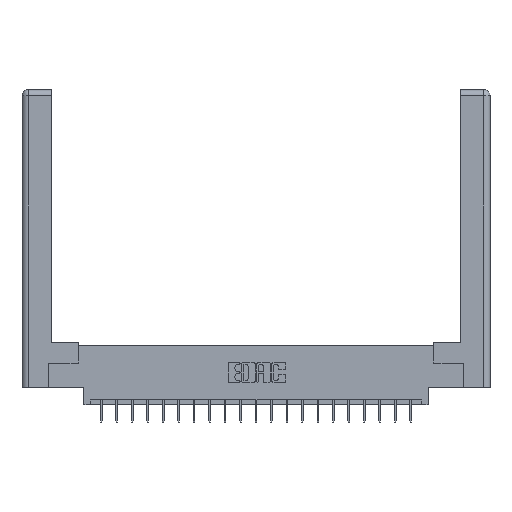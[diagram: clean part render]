
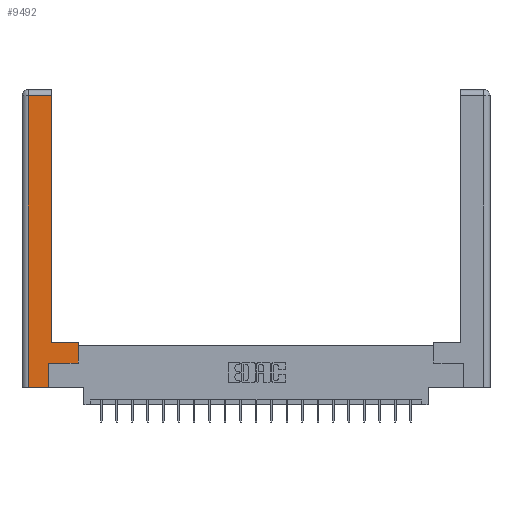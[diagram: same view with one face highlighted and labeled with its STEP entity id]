
A CAD part, top view. The second image highlights one B-rep face of the part: STEP entity #9492.
In plain terms, the highlighted planar face has unit normal (0, 0, 1).
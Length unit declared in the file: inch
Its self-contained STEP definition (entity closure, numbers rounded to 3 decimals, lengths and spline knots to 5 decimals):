
#692 = ORIENTED_EDGE ( 'NONE', *, *, #14860, .T. ) ;
#782 = EDGE_LOOP ( 'NONE', ( #16485, #2539, #20749, #16274, #4995, #19639, #21707, #692 ) ) ;
#1170 = VECTOR ( 'NONE', #1646, 39.37008 ) ;
#1510 = DIRECTION ( 'NONE',  ( 0., 1., 0. ) ) ;
#1646 = DIRECTION ( 'NONE',  ( 0., 1., 0. ) ) ;
#2276 = CARTESIAN_POINT ( 'NONE',  ( 0.565, 0.45, 0. ) ) ;
#2539 = ORIENTED_EDGE ( 'NONE', *, *, #13917, .T. ) ;
#2809 = EDGE_CURVE ( 'NONE', #17671, #3995, #18349, .T. ) ;
#3052 = CARTESIAN_POINT ( 'NONE',  ( 0.565, 0.45, 0. ) ) ;
#3995 = VERTEX_POINT ( 'NONE', #11574 ) ;
#4002 = DIRECTION ( 'NONE',  ( 1., 0., 0. ) ) ;
#4779 = EDGE_CURVE ( 'NONE', #21580, #12341, #20707, .T. ) ;
#4995 = ORIENTED_EDGE ( 'NONE', *, *, #2809, .T. ) ;
#5110 = VERTEX_POINT ( 'NONE', #9535 ) ;
#6011 = CARTESIAN_POINT ( 'NONE',  ( 0., 0., 0. ) ) ;
#6111 = CARTESIAN_POINT ( 'NONE',  ( 0.265, 0.245, 0. ) ) ;
#6197 = CARTESIAN_POINT ( 'NONE',  ( 0.0615, 2.94, 0. ) ) ;
#7934 = DIRECTION ( 'NONE',  ( 0., 1., 0. ) ) ;
#8126 = VERTEX_POINT ( 'NONE', #19199 ) ;
#8534 = LINE ( 'NONE', #13625, #19626 ) ;
#8620 = FACE_OUTER_BOUND ( 'NONE', #782, .T. ) ;
#9492 = ADVANCED_FACE ( 'NONE', ( #8620 ), #19507, .F. ) ;
#9535 = CARTESIAN_POINT ( 'NONE',  ( 0.295, 0.45, 0. ) ) ;
#10474 = VECTOR ( 'NONE', #17544, 39.37008 ) ;
#10750 = LINE ( 'NONE', #17470, #10474 ) ;
#11574 = CARTESIAN_POINT ( 'NONE',  ( 0.265, 0.245, 0. ) ) ;
#11628 = CARTESIAN_POINT ( 'NONE',  ( 0.295, 3., 0. ) ) ;
#11788 = VERTEX_POINT ( 'NONE', #6197 ) ;
#12341 = VERTEX_POINT ( 'NONE', #2276 ) ;
#12623 = VECTOR ( 'NONE', #17944, 39.37008 ) ;
#13130 = VECTOR ( 'NONE', #1510, 39.37008 ) ;
#13625 = CARTESIAN_POINT ( 'NONE',  ( 0.295, 0.45, 0. ) ) ;
#13877 = VECTOR ( 'NONE', #7934, 39.37008 ) ;
#13917 = EDGE_CURVE ( 'NONE', #18769, #11788, #18325, .T. ) ;
#14104 = CARTESIAN_POINT ( 'NONE',  ( 0.0615, 0., 0. ) ) ;
#14414 = AXIS2_PLACEMENT_3D ( 'NONE', #6011, #15960, #16260 ) ;
#14810 = DIRECTION ( 'NONE',  ( -1., 0., 0. ) ) ;
#14860 = EDGE_CURVE ( 'NONE', #12341, #5110, #8534, .T. ) ;
#15720 = VECTOR ( 'NONE', #14810, 39.37008 ) ;
#15960 = DIRECTION ( 'NONE',  ( 0., 0., -1. ) ) ;
#16260 = DIRECTION ( 'NONE',  ( -1., 0., 0. ) ) ;
#16274 = ORIENTED_EDGE ( 'NONE', *, *, #21083, .T. ) ;
#16485 = ORIENTED_EDGE ( 'NONE', *, *, #20163, .T. ) ;
#17470 = CARTESIAN_POINT ( 'NONE',  ( 0.265, 0., 0. ) ) ;
#17544 = DIRECTION ( 'NONE',  ( 1., 0., 0. ) ) ;
#17558 = CARTESIAN_POINT ( 'NONE',  ( 0.565, 0.245, 0. ) ) ;
#17570 = CARTESIAN_POINT ( 'NONE',  ( 0.565, 0.245, 0. ) ) ;
#17671 = VERTEX_POINT ( 'NONE', #18362 ) ;
#17944 = DIRECTION ( 'NONE',  ( 0., -1., 0. ) ) ;
#17969 = EDGE_CURVE ( 'NONE', #3995, #21580, #18474, .T. ) ;
#18124 = CARTESIAN_POINT ( 'NONE',  ( 0.295, 2.94, 0. ) ) ;
#18163 = LINE ( 'NONE', #14104, #12623 ) ;
#18325 = LINE ( 'NONE', #21716, #15720 ) ;
#18349 = LINE ( 'NONE', #6111, #13877 ) ;
#18362 = CARTESIAN_POINT ( 'NONE',  ( 0.265, 0., 0. ) ) ;
#18474 = LINE ( 'NONE', #17558, #20334 ) ;
#18769 = VERTEX_POINT ( 'NONE', #18124 ) ;
#19049 = EDGE_CURVE ( 'NONE', #11788, #8126, #18163, .T. ) ;
#19199 = CARTESIAN_POINT ( 'NONE',  ( 0.0615, 0., 0. ) ) ;
#19507 = PLANE ( 'NONE',  #14414 ) ;
#19626 = VECTOR ( 'NONE', #20414, 39.37008 ) ;
#19639 = ORIENTED_EDGE ( 'NONE', *, *, #17969, .T. ) ;
#20163 = EDGE_CURVE ( 'NONE', #5110, #18769, #20802, .T. ) ;
#20334 = VECTOR ( 'NONE', #4002, 39.37008 ) ;
#20414 = DIRECTION ( 'NONE',  ( -1., 0., 0. ) ) ;
#20707 = LINE ( 'NONE', #3052, #1170 ) ;
#20749 = ORIENTED_EDGE ( 'NONE', *, *, #19049, .T. ) ;
#20802 = LINE ( 'NONE', #11628, #13130 ) ;
#21083 = EDGE_CURVE ( 'NONE', #8126, #17671, #10750, .T. ) ;
#21580 = VERTEX_POINT ( 'NONE', #17570 ) ;
#21707 = ORIENTED_EDGE ( 'NONE', *, *, #4779, .T. ) ;
#21716 = CARTESIAN_POINT ( 'NONE',  ( 0.0615, 2.94, 0. ) ) ;
